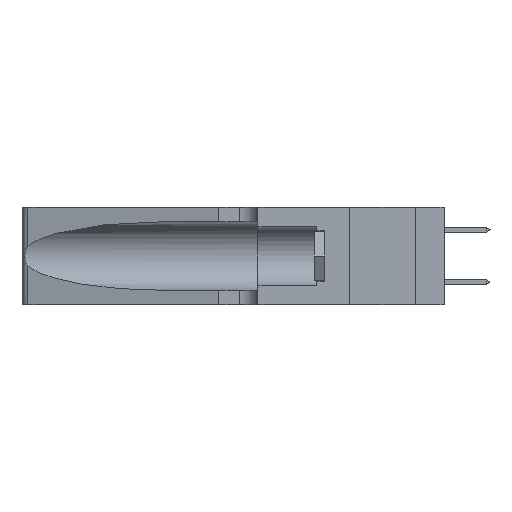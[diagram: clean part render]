
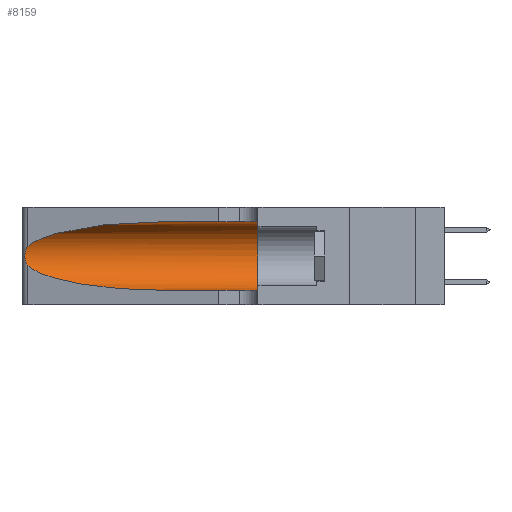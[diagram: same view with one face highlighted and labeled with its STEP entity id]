
A CAD part, left-side view. The second image highlights one B-rep face of the part: STEP entity #8159.
In plain terms, the highlighted cylindrical face has radius 3.308 mm (diameter 6.617 mm), a partial arc.
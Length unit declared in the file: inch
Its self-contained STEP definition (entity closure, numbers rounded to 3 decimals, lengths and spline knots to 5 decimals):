
#1036 = EDGE_CURVE ( 'NONE', #14686, #14479, #22632, .T. ) ;
#1426 = CARTESIAN_POINT ( 'NONE',  ( 0.2373, 1.15595, 0.08982 ) ) ;
#1990 = AXIS2_PLACEMENT_3D ( 'NONE', #18749, #2397, #8016 ) ;
#2397 = DIRECTION ( 'NONE',  ( 0., 1., 0. ) ) ;
#3485 = ORIENTED_EDGE ( 'NONE', *, *, #1036, .T. ) ;
#3767 = CARTESIAN_POINT ( 'NONE',  ( 0.25555, 1.22994, 0.2215 ) ) ;
#5574 = CARTESIAN_POINT ( 'NONE',  ( 0.25487, 1.22718, 0.14631 ) ) ;
#6043 = VECTOR ( 'NONE', #31750, 39.37008 ) ;
#6108 = ORIENTED_EDGE ( 'NONE', *, *, #13008, .T. ) ;
#6195 = VERTEX_POINT ( 'NONE', #31852 ) ;
#6443 = CARTESIAN_POINT ( 'NONE',  ( 0.1305, 0.72297, 0.31525 ) ) ;
#6670 = LINE ( 'NONE', #27476, #26729 ) ;
#6720 = B_SPLINE_CURVE_WITH_KNOTS ( 'NONE', 3,
 ( #33720, #3767, #19964, #11880, #9130, #9375, #11997, #6739, #6855, #31447, #14735, #28580, #17474, #30990 ),
 .UNSPECIFIED., .F., .F.,
 ( 4, 2, 2, 2, 2, 2, 4 ),
 ( 0., 0.00027, 0.00053, 0.00107, 0.0016, 0.00187, 0.00214 ),
 .UNSPECIFIED. ) ;
#6739 = CARTESIAN_POINT ( 'NONE',  ( 0.26075, 1.23896, 0.178 ) ) ;
#6855 = CARTESIAN_POINT ( 'NONE',  ( 0.26017, 1.23833, 0.17102 ) ) ;
#7237 = AXIS2_PLACEMENT_3D ( 'NONE', #34802, #8181, #14029 ) ;
#7519 = CARTESIAN_POINT ( 'NONE',  ( 0.1305, 0.35, 0.31525 ) ) ;
#7796 =( BOUNDED_CURVE ( )  B_SPLINE_CURVE ( 3, ( #6443, #15135, #10344, #12610 ),
 .UNSPECIFIED., .F., .T. ) 
 B_SPLINE_CURVE_WITH_KNOTS ( ( 4, 4 ),
 ( 1.5708, 2.84003 ),
 .UNSPECIFIED. ) 
 CURVE ( )  GEOMETRIC_REPRESENTATION_ITEM ( )  RATIONAL_B_SPLINE_CURVE ( ( 1., 0.87, 0.87, 1. ) ) 
 REPRESENTATION_ITEM ( '' )  );
#8016 = DIRECTION ( 'NONE',  ( 0., 0., 1. ) ) ;
#8159 = ADVANCED_FACE ( 'NONE', ( #15708 ), #8458, .F. ) ;
#8181 = DIRECTION ( 'NONE',  ( 0., -1., 0. ) ) ;
#8458 = CYLINDRICAL_SURFACE ( 'NONE', #7237, 0.13025 ) ;
#9130 = CARTESIAN_POINT ( 'NONE',  ( 0.25854, 1.2359, 0.20912 ) ) ;
#9312 = EDGE_CURVE ( 'NONE', #14479, #18318, #6670, .T. ) ;
#9375 = CARTESIAN_POINT ( 'NONE',  ( 0.26018, 1.23835, 0.19895 ) ) ;
#10018 = EDGE_CURVE ( 'NONE', #6195, #16355, #7796, .T. ) ;
#10344 = CARTESIAN_POINT ( 'NONE',  ( 0.2373, 1.15595, 0.28018 ) ) ;
#10868 = ORIENTED_EDGE ( 'NONE', *, *, #18076, .F. ) ;
#11696 = CARTESIAN_POINT ( 'NONE',  ( 0.25487, 1.22718, 0.22369 ) ) ;
#11880 = CARTESIAN_POINT ( 'NONE',  ( 0.25787, 1.23484, 0.2124 ) ) ;
#11997 = CARTESIAN_POINT ( 'NONE',  ( 0.26075, 1.23896, 0.19203 ) ) ;
#12114 = EDGE_LOOP ( 'NONE', ( #23656, #6108, #3485, #28753, #10868, #34777 ) ) ;
#12610 = CARTESIAN_POINT ( 'NONE',  ( 0.25487, 1.22718, 0.22369 ) ) ;
#13008 = EDGE_CURVE ( 'NONE', #16355, #14686, #6720, .T. ) ;
#14029 = DIRECTION ( 'NONE',  ( 0., 0., -1. ) ) ;
#14479 = VERTEX_POINT ( 'NONE', #25988 ) ;
#14686 = VERTEX_POINT ( 'NONE', #5574 ) ;
#14735 = CARTESIAN_POINT ( 'NONE',  ( 0.25789, 1.23486, 0.15765 ) ) ;
#14933 = CARTESIAN_POINT ( 'NONE',  ( 0.25487, 1.22718, 0.14631 ) ) ;
#15135 = CARTESIAN_POINT ( 'NONE',  ( 0.18966, 0.96281, 0.31525 ) ) ;
#15708 = FACE_OUTER_BOUND ( 'NONE', #12114, .T. ) ;
#16355 = VERTEX_POINT ( 'NONE', #11696 ) ;
#17474 = CARTESIAN_POINT ( 'NONE',  ( 0.25555, 1.22993, 0.14849 ) ) ;
#18076 = EDGE_CURVE ( 'NONE', #24369, #18318, #29112, .T. ) ;
#18318 = VERTEX_POINT ( 'NONE', #22754 ) ;
#18535 = EDGE_CURVE ( 'NONE', #6195, #24369, #22219, .T. ) ;
#18749 = CARTESIAN_POINT ( 'NONE',  ( 0.1305, 0.35, 0.185 ) ) ;
#19964 = CARTESIAN_POINT ( 'NONE',  ( 0.25639, 1.23184, 0.21858 ) ) ;
#22219 = LINE ( 'NONE', #28989, #6043 ) ;
#22632 =( BOUNDED_CURVE ( )  B_SPLINE_CURVE ( 3, ( #14933, #1426, #26042, #29612 ),
 .UNSPECIFIED., .F., .F. ) 
 B_SPLINE_CURVE_WITH_KNOTS ( ( 4, 4 ),
 ( 3.44316, 4.71239 ),
 .UNSPECIFIED. ) 
 CURVE ( )  GEOMETRIC_REPRESENTATION_ITEM ( )  RATIONAL_B_SPLINE_CURVE ( ( 1., 0.87, 0.87, 1. ) ) 
 REPRESENTATION_ITEM ( '' )  );
#22754 = CARTESIAN_POINT ( 'NONE',  ( 0.1305, 0.35, 0.05475 ) ) ;
#23656 = ORIENTED_EDGE ( 'NONE', *, *, #10018, .T. ) ;
#24369 = VERTEX_POINT ( 'NONE', #7519 ) ;
#25988 = CARTESIAN_POINT ( 'NONE',  ( 0.1305, 0.72297, 0.05475 ) ) ;
#26042 = CARTESIAN_POINT ( 'NONE',  ( 0.18966, 0.96281, 0.05475 ) ) ;
#26729 = VECTOR ( 'NONE', #27241, 39.37008 ) ;
#27241 = DIRECTION ( 'NONE',  ( 0., -1., 0. ) ) ;
#27476 = CARTESIAN_POINT ( 'NONE',  ( 0.1305, 1.61858, 0.05475 ) ) ;
#28580 = CARTESIAN_POINT ( 'NONE',  ( 0.25639, 1.23186, 0.15144 ) ) ;
#28753 = ORIENTED_EDGE ( 'NONE', *, *, #9312, .T. ) ;
#28989 = CARTESIAN_POINT ( 'NONE',  ( 0.1305, 1.61858, 0.31525 ) ) ;
#29112 = CIRCLE ( 'NONE', #1990, 0.13025 ) ;
#29612 = CARTESIAN_POINT ( 'NONE',  ( 0.1305, 0.72297, 0.05475 ) ) ;
#30990 = CARTESIAN_POINT ( 'NONE',  ( 0.25487, 1.22718, 0.14631 ) ) ;
#31447 = CARTESIAN_POINT ( 'NONE',  ( 0.25856, 1.23593, 0.16098 ) ) ;
#31750 = DIRECTION ( 'NONE',  ( 0., -1., 0. ) ) ;
#31852 = CARTESIAN_POINT ( 'NONE',  ( 0.1305, 0.72297, 0.31525 ) ) ;
#33720 = CARTESIAN_POINT ( 'NONE',  ( 0.25487, 1.22718, 0.22369 ) ) ;
#34777 = ORIENTED_EDGE ( 'NONE', *, *, #18535, .F. ) ;
#34802 = CARTESIAN_POINT ( 'NONE',  ( 0.1305, 1.61858, 0.185 ) ) ;
